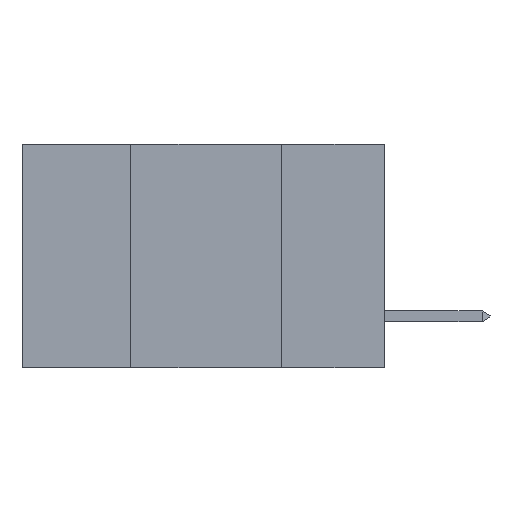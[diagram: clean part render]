
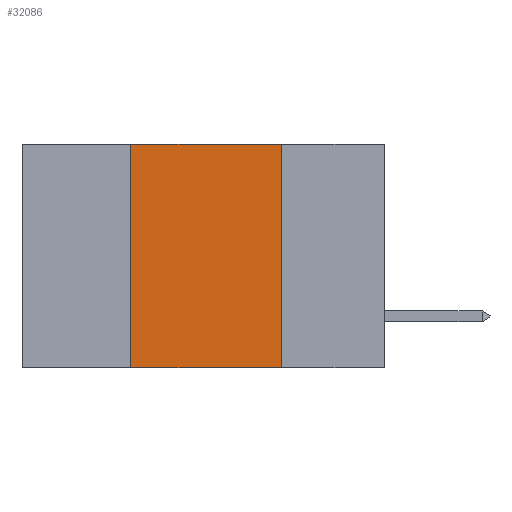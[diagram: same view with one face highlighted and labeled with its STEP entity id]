
A CAD part, left-side view. The second image highlights one B-rep face of the part: STEP entity #32086.
In plain terms, the highlighted planar face has unit normal (-1, 0, 0).
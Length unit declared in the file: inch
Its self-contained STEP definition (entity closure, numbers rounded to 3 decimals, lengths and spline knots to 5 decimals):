
#523 = VECTOR ( 'NONE', #30148, 39.37008 ) ;
#811 = EDGE_CURVE ( 'NONE', #22256, #37022, #32872, .T. ) ;
#2105 = DIRECTION ( 'NONE',  ( 0., 0., -1. ) ) ;
#2574 = CARTESIAN_POINT ( 'NONE',  ( 0., 0.42, -0.37 ) ) ;
#2787 = CARTESIAN_POINT ( 'NONE',  ( 0., 0.6, -0.37 ) ) ;
#3375 = CARTESIAN_POINT ( 'NONE',  ( 0., 0.6, 0. ) ) ;
#3996 = FACE_OUTER_BOUND ( 'NONE', #22286, .T. ) ;
#5229 = VECTOR ( 'NONE', #2105, 39.37008 ) ;
#6666 = LINE ( 'NONE', #3375, #523 ) ;
#10362 = CARTESIAN_POINT ( 'NONE',  ( 0., 0.6, 0. ) ) ;
#10556 = CARTESIAN_POINT ( 'NONE',  ( 0., 0.17, -0.37 ) ) ;
#10851 = ORIENTED_EDGE ( 'NONE', *, *, #22898, .F. ) ;
#11393 = ORIENTED_EDGE ( 'NONE', *, *, #17308, .F. ) ;
#12006 = VECTOR ( 'NONE', #24643, 39.37008 ) ;
#12285 = VERTEX_POINT ( 'NONE', #41580 ) ;
#12673 = ORIENTED_EDGE ( 'NONE', *, *, #811, .T. ) ;
#13097 = EDGE_CURVE ( 'NONE', #12285, #37022, #18574, .T. ) ;
#13114 = DIRECTION ( 'NONE',  ( 0., -1., 0. ) ) ;
#13523 = VECTOR ( 'NONE', #13114, 39.37008 ) ;
#17308 = EDGE_CURVE ( 'NONE', #36701, #12285, #6666, .T. ) ;
#18574 = LINE ( 'NONE', #35260, #5229 ) ;
#20225 = PLANE ( 'NONE',  #43002 ) ;
#22256 = VERTEX_POINT ( 'NONE', #2574 ) ;
#22286 = EDGE_LOOP ( 'NONE', ( #22523, #11393, #10851, #12673 ) ) ;
#22523 = ORIENTED_EDGE ( 'NONE', *, *, #13097, .F. ) ;
#22898 = EDGE_CURVE ( 'NONE', #22256, #36701, #37186, .T. ) ;
#24643 = DIRECTION ( 'NONE',  ( 0., 0., 1. ) ) ;
#27518 = CARTESIAN_POINT ( 'NONE',  ( 0., 0.42, 0. ) ) ;
#27792 = CARTESIAN_POINT ( 'NONE',  ( 0., 0.42, 0. ) ) ;
#30148 = DIRECTION ( 'NONE',  ( 0., -1., 0. ) ) ;
#32086 = ADVANCED_FACE ( 'NONE', ( #3996 ), #20225, .F. ) ;
#32872 = LINE ( 'NONE', #2787, #13523 ) ;
#35260 = CARTESIAN_POINT ( 'NONE',  ( 0., 0.17, 0. ) ) ;
#36701 = VERTEX_POINT ( 'NONE', #27792 ) ;
#36705 = DIRECTION ( 'NONE',  ( 0., 0., -1. ) ) ;
#37022 = VERTEX_POINT ( 'NONE', #10556 ) ;
#37147 = DIRECTION ( 'NONE',  ( 1., 0., 0. ) ) ;
#37186 = LINE ( 'NONE', #27518, #12006 ) ;
#41580 = CARTESIAN_POINT ( 'NONE',  ( 0., 0.17, 0. ) ) ;
#43002 = AXIS2_PLACEMENT_3D ( 'NONE', #10362, #37147, #36705 ) ;
